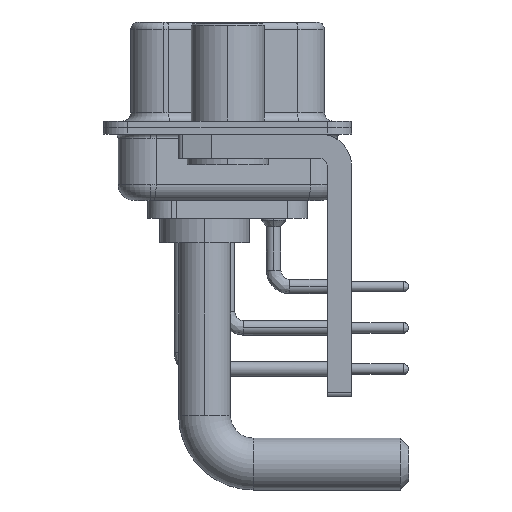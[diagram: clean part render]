
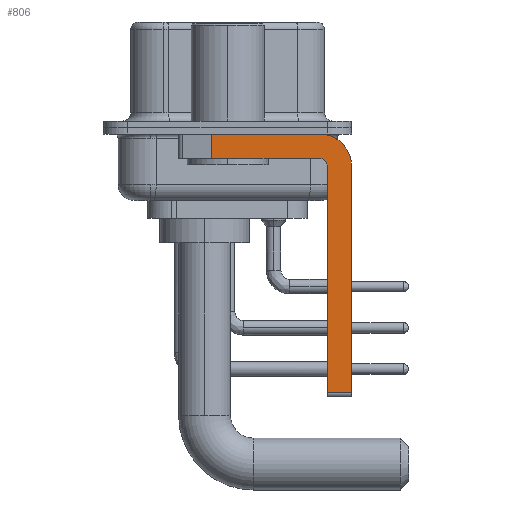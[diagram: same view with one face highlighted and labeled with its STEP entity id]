
A CAD part, left-side view. The second image highlights one B-rep face of the part: STEP entity #806.
In plain terms, the highlighted planar face has unit normal (-1, 0, 0).
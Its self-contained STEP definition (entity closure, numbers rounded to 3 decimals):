
#281 = EDGE_CURVE ( 'NONE', #8657, #11593, #19377, .T. ) ;
#506 = EDGE_CURVE ( 'NONE', #16307, #8657, #36376, .T. ) ;
#541 = DIRECTION ( 'NONE',  ( 1., 0., 0. ) ) ;
#715 = CARTESIAN_POINT ( 'NONE',  ( -2.9, -5.65, -2.4 ) ) ;
#806 = ADVANCED_FACE ( 'NONE', ( #9824 ), #20773, .F. ) ;
#833 = VERTEX_POINT ( 'NONE', #20399 ) ;
#997 = CARTESIAN_POINT ( 'NONE',  ( -2.9, -5.65, -16.35 ) ) ;
#1314 = CIRCLE ( 'NONE', #20872, 2. ) ;
#2971 = CARTESIAN_POINT ( 'NONE',  ( -2.9, 0.978, -1.9 ) ) ;
#3712 = ORIENTED_EDGE ( 'NONE', *, *, #27755, .T. ) ;
#3910 = EDGE_CURVE ( 'NONE', #833, #16593, #22996, .T. ) ;
#4392 = AXIS2_PLACEMENT_3D ( 'NONE', #715, #541, #9102 ) ;
#4720 = CARTESIAN_POINT ( 'NONE',  ( -2.9, 0.978, -1.9 ) ) ;
#5429 = ORIENTED_EDGE ( 'NONE', *, *, #3910, .F. ) ;
#5781 = VECTOR ( 'NONE', #34795, 1000. ) ;
#5882 = CARTESIAN_POINT ( 'NONE',  ( -2.9, 3., -0.4 ) ) ;
#6911 = CARTESIAN_POINT ( 'NONE',  ( -2.9, -5.65, -0.4 ) ) ;
#7820 = CARTESIAN_POINT ( 'NONE',  ( -2.9, -7.65, -16.35 ) ) ;
#8657 = VERTEX_POINT ( 'NONE', #28377 ) ;
#8872 = LINE ( 'NONE', #997, #10618 ) ;
#9102 = DIRECTION ( 'NONE',  ( 0., 0., -1. ) ) ;
#9362 = CARTESIAN_POINT ( 'NONE',  ( -2.9, -6.15, -16.6 ) ) ;
#9658 = ORIENTED_EDGE ( 'NONE', *, *, #281, .F. ) ;
#9824 = FACE_OUTER_BOUND ( 'NONE', #23128, .T. ) ;
#10290 = LINE ( 'NONE', #4720, #21781 ) ;
#10618 = VECTOR ( 'NONE', #23654, 1000. ) ;
#11265 = LINE ( 'NONE', #5882, #16075 ) ;
#11593 = VERTEX_POINT ( 'NONE', #2971 ) ;
#12123 = VERTEX_POINT ( 'NONE', #14231 ) ;
#12698 = EDGE_CURVE ( 'NONE', #12123, #16307, #31458, .T. ) ;
#12975 = DIRECTION ( 'NONE',  ( 0., 0., -1. ) ) ;
#14231 = CARTESIAN_POINT ( 'NONE',  ( -2.9, -6.15, -16.35 ) ) ;
#14882 = CARTESIAN_POINT ( 'NONE',  ( -2.9, -6.15, -2.4 ) ) ;
#15827 = VECTOR ( 'NONE', #31339, 1000. ) ;
#15952 = EDGE_CURVE ( 'NONE', #12123, #16593, #8872, .T. ) ;
#16035 = DIRECTION ( 'NONE',  ( 0., 0., -1. ) ) ;
#16075 = VECTOR ( 'NONE', #28881, 1000. ) ;
#16307 = VERTEX_POINT ( 'NONE', #14882 ) ;
#16593 = VERTEX_POINT ( 'NONE', #7820 ) ;
#17963 = EDGE_CURVE ( 'NONE', #34022, #28026, #11265, .T. ) ;
#19377 = LINE ( 'NONE', #27742, #24491 ) ;
#20381 = CARTESIAN_POINT ( 'NONE',  ( -2.9, -7.65, -2.4 ) ) ;
#20399 = CARTESIAN_POINT ( 'NONE',  ( -2.9, -7.65, -2.4 ) ) ;
#20547 = ORIENTED_EDGE ( 'NONE', *, *, #17963, .F. ) ;
#20773 = PLANE ( 'NONE',  #4392 ) ;
#20872 = AXIS2_PLACEMENT_3D ( 'NONE', #26723, #32301, #12975 ) ;
#21230 = DIRECTION ( 'NONE',  ( -1., 0., 0. ) ) ;
#21781 = VECTOR ( 'NONE', #16035, 1000. ) ;
#22552 = DIRECTION ( 'NONE',  ( 0., 1., 0. ) ) ;
#22996 = LINE ( 'NONE', #20381, #15827 ) ;
#23128 = EDGE_LOOP ( 'NONE', ( #20547, #3712, #9658, #36437, #36148, #36196, #5429, #33407 ) ) ;
#23654 = DIRECTION ( 'NONE',  ( 0., -1., 0. ) ) ;
#24491 = VECTOR ( 'NONE', #22552, 1000. ) ;
#24693 = CARTESIAN_POINT ( 'NONE',  ( -2.9, 0.978, -0.4 ) ) ;
#26723 = CARTESIAN_POINT ( 'NONE',  ( -2.9, -5.65, -2.4 ) ) ;
#27457 = DIRECTION ( 'NONE',  ( 0., 0., 1. ) ) ;
#27742 = CARTESIAN_POINT ( 'NONE',  ( -2.9, -5.65, -1.9 ) ) ;
#27755 = EDGE_CURVE ( 'NONE', #34022, #11593, #10290, .T. ) ;
#28026 = VERTEX_POINT ( 'NONE', #6911 ) ;
#28056 = AXIS2_PLACEMENT_3D ( 'NONE', #35354, #21230, #27457 ) ;
#28377 = CARTESIAN_POINT ( 'NONE',  ( -2.9, -5.65, -1.9 ) ) ;
#28881 = DIRECTION ( 'NONE',  ( 0., -1., 0. ) ) ;
#31339 = DIRECTION ( 'NONE',  ( 0., 0., -1. ) ) ;
#31458 = LINE ( 'NONE', #9362, #5781 ) ;
#32301 = DIRECTION ( 'NONE',  ( 1., 0., 0. ) ) ;
#33407 = ORIENTED_EDGE ( 'NONE', *, *, #35650, .F. ) ;
#34022 = VERTEX_POINT ( 'NONE', #24693 ) ;
#34795 = DIRECTION ( 'NONE',  ( 0., 0., 1. ) ) ;
#35354 = CARTESIAN_POINT ( 'NONE',  ( -2.9, -5.65, -2.4 ) ) ;
#35650 = EDGE_CURVE ( 'NONE', #28026, #833, #1314, .T. ) ;
#36148 = ORIENTED_EDGE ( 'NONE', *, *, #12698, .F. ) ;
#36196 = ORIENTED_EDGE ( 'NONE', *, *, #15952, .T. ) ;
#36376 = CIRCLE ( 'NONE', #28056, 0.5 ) ;
#36437 = ORIENTED_EDGE ( 'NONE', *, *, #506, .F. ) ;
